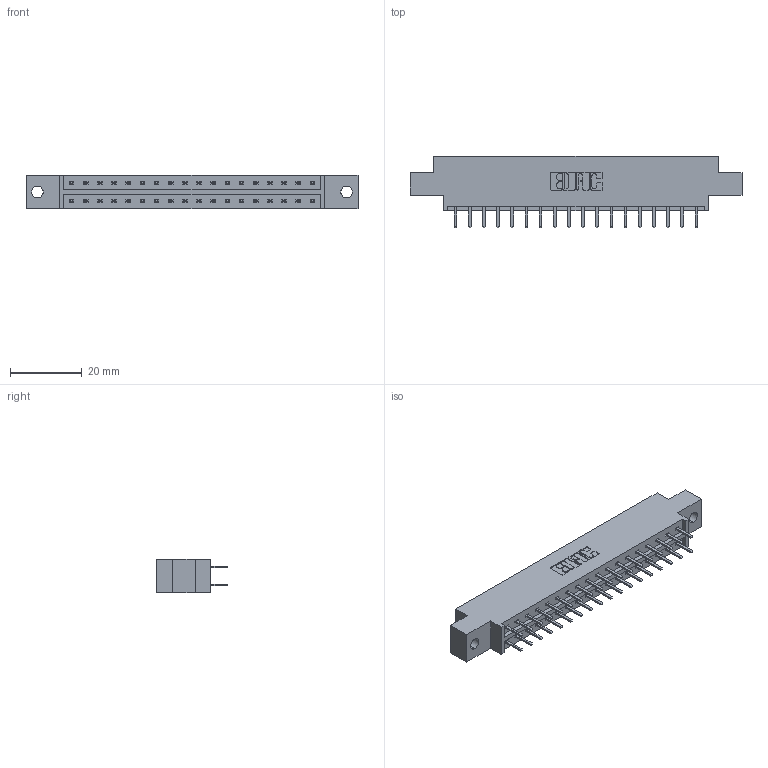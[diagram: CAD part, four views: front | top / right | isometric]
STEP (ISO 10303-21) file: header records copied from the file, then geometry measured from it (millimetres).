
FILE_DESCRIPTION (( 'STEP AP203' ), '1' );
FILE_NAME ('833-036-520-802.STEP', '2020-06-03T01:45:56', ( '' ), ( '' ), 'SwSTEP 2.0', 'SolidWorks 2020', '' );
FILE_SCHEMA (( 'CONFIG_CONTROL_DESIGN' ));
Length unit declared in the file: inch
Products named in the file (3): 833-036-520-802; 833 Part_Offset - .128 Dia; 345-292-001_345-293-120
Assembly tree (37 placements, depth 2):
  833-036-520-802
    833 Part_Offset - .128 Dia
    345-292-001_345-293-120  x36
Bounding box: 92.86 x 20.02 x 9.4 mm (x, y, z)
Volume: 8976 mm3; surface area: 10259.5 mm2
Topology: 37 solids, 37 shells, 2134 faces, 6191 edges, 4030 vertices
Faces by surface type: plane 1442, cylinder 692
Entity records: 14933 total; most frequent: CARTESIAN_POINT 2518, ORIENTED_EDGE 2442, DIRECTION 2181, EDGE_CURVE 1221, VECTOR 1089, LINE 1089, VERTEX_POINT 810, AXIS2_PLACEMENT_3D 546
